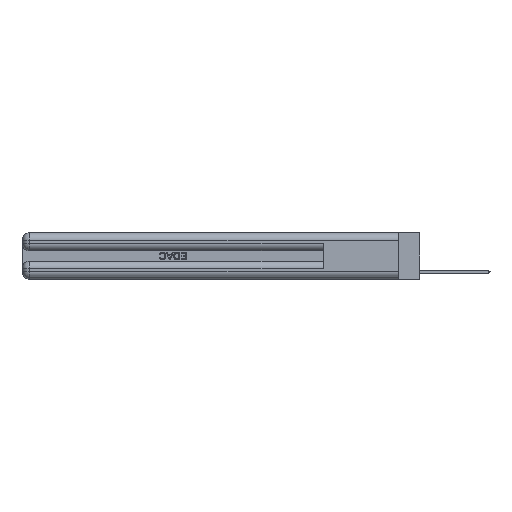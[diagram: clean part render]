
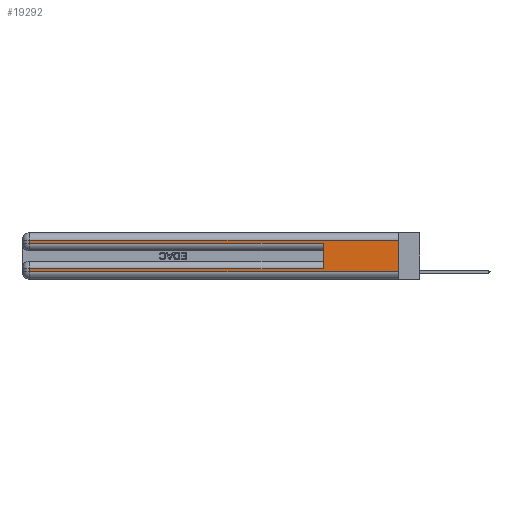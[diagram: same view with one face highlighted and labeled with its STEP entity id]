
A CAD part, left-side view. The second image highlights one B-rep face of the part: STEP entity #19292.
In plain terms, the highlighted planar face has unit normal (-1, 0, 0).
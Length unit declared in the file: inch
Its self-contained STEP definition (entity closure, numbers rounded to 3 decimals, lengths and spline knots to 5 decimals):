
#605 = VERTEX_POINT ( 'NONE', #7229 ) ;
#1070 = VECTOR ( 'NONE', #4378, 39.37008 ) ;
#1285 = LINE ( 'NONE', #17142, #4442 ) ;
#1481 = CARTESIAN_POINT ( 'NONE',  ( 0., 0.6, 0.145 ) ) ;
#1705 = CARTESIAN_POINT ( 'NONE',  ( 0., 0., 0.285 ) ) ;
#2205 = DIRECTION ( 'NONE',  ( 0., -1., 0. ) ) ;
#2462 = DIRECTION ( 'NONE',  ( 0., 0., 1. ) ) ;
#2472 = CARTESIAN_POINT ( 'NONE',  ( 0., 0., 0.31 ) ) ;
#3097 = VERTEX_POINT ( 'NONE', #30010 ) ;
#3141 = EDGE_CURVE ( 'NONE', #605, #27301, #4710, .T. ) ;
#3662 = ORIENTED_EDGE ( 'NONE', *, *, #11765, .T. ) ;
#3922 = CARTESIAN_POINT ( 'NONE',  ( 0., 2.94, 0.085 ) ) ;
#4378 = DIRECTION ( 'NONE',  ( 0., 1., 0. ) ) ;
#4442 = VECTOR ( 'NONE', #14742, 39.37008 ) ;
#4710 = LINE ( 'NONE', #27441, #1070 ) ;
#5021 = DIRECTION ( 'NONE',  ( 0., 1., 0. ) ) ;
#6286 = CARTESIAN_POINT ( 'NONE',  ( 0., 0., 0.37 ) ) ;
#6778 = VERTEX_POINT ( 'NONE', #8180 ) ;
#7229 = CARTESIAN_POINT ( 'NONE',  ( 0., 0.6, 0.085 ) ) ;
#7484 = AXIS2_PLACEMENT_3D ( 'NONE', #27236, #9114, #19537 ) ;
#7541 = ORIENTED_EDGE ( 'NONE', *, *, #27894, .T. ) ;
#7561 = LINE ( 'NONE', #2472, #8804 ) ;
#8180 = CARTESIAN_POINT ( 'NONE',  ( 0., 2.94, 0.285 ) ) ;
#8693 = CARTESIAN_POINT ( 'NONE',  ( 0., 0.6, 0.285 ) ) ;
#8804 = VECTOR ( 'NONE', #5021, 39.37008 ) ;
#9114 = DIRECTION ( 'NONE',  ( 1., 0., 0. ) ) ;
#9680 = VECTOR ( 'NONE', #14463, 39.37008 ) ;
#10110 = ORIENTED_EDGE ( 'NONE', *, *, #33695, .T. ) ;
#10632 = ORIENTED_EDGE ( 'NONE', *, *, #3141, .T. ) ;
#11725 = VERTEX_POINT ( 'NONE', #26960 ) ;
#11765 = EDGE_CURVE ( 'NONE', #28287, #6778, #12047, .T. ) ;
#12047 = LINE ( 'NONE', #19926, #14312 ) ;
#12057 = VERTEX_POINT ( 'NONE', #29638 ) ;
#12223 = DIRECTION ( 'NONE',  ( 0., 0., -1. ) ) ;
#12850 = VECTOR ( 'NONE', #2462, 39.37008 ) ;
#14312 = VECTOR ( 'NONE', #12223, 39.37008 ) ;
#14463 = DIRECTION ( 'NONE',  ( 0., 0., -1. ) ) ;
#14520 = VECTOR ( 'NONE', #2205, 39.37008 ) ;
#14742 = DIRECTION ( 'NONE',  ( 0., 0., -1. ) ) ;
#14872 = CARTESIAN_POINT ( 'NONE',  ( 0., 0., 0.06 ) ) ;
#14916 = PLANE ( 'NONE',  #7484 ) ;
#16235 = VECTOR ( 'NONE', #32496, 39.37008 ) ;
#17142 = CARTESIAN_POINT ( 'NONE',  ( 0., 2.94, 0.37 ) ) ;
#17559 = EDGE_CURVE ( 'NONE', #605, #18305, #29842, .T. ) ;
#17745 = LINE ( 'NONE', #1705, #14520 ) ;
#18138 = CARTESIAN_POINT ( 'NONE',  ( 0., 2.94, 0.31 ) ) ;
#18305 = VERTEX_POINT ( 'NONE', #8693 ) ;
#18437 = EDGE_CURVE ( 'NONE', #6778, #18305, #17745, .T. ) ;
#19088 = EDGE_LOOP ( 'NONE', ( #21956, #7541, #3662, #22763, #26544, #10632, #31064, #10110 ) ) ;
#19292 = ADVANCED_FACE ( 'NONE', ( #22783 ), #14916, .F. ) ;
#19537 = DIRECTION ( 'NONE',  ( 0., 0., -1. ) ) ;
#19926 = CARTESIAN_POINT ( 'NONE',  ( 0., 2.94, 0.37 ) ) ;
#21587 = EDGE_CURVE ( 'NONE', #12057, #11725, #27473, .T. ) ;
#21956 = ORIENTED_EDGE ( 'NONE', *, *, #21587, .F. ) ;
#22763 = ORIENTED_EDGE ( 'NONE', *, *, #18437, .T. ) ;
#22783 = FACE_OUTER_BOUND ( 'NONE', #19088, .T. ) ;
#24970 = LINE ( 'NONE', #14872, #16235 ) ;
#26544 = ORIENTED_EDGE ( 'NONE', *, *, #17559, .F. ) ;
#26960 = CARTESIAN_POINT ( 'NONE',  ( 0., 0., 0.06 ) ) ;
#27236 = CARTESIAN_POINT ( 'NONE',  ( 0., 0., 0.37 ) ) ;
#27301 = VERTEX_POINT ( 'NONE', #3922 ) ;
#27441 = CARTESIAN_POINT ( 'NONE',  ( 0., 0., 0.085 ) ) ;
#27473 = LINE ( 'NONE', #6286, #9680 ) ;
#27691 = EDGE_CURVE ( 'NONE', #27301, #3097, #1285, .T. ) ;
#27894 = EDGE_CURVE ( 'NONE', #12057, #28287, #7561, .T. ) ;
#28287 = VERTEX_POINT ( 'NONE', #18138 ) ;
#29638 = CARTESIAN_POINT ( 'NONE',  ( 0., 0., 0.31 ) ) ;
#29842 = LINE ( 'NONE', #1481, #12850 ) ;
#30010 = CARTESIAN_POINT ( 'NONE',  ( 0., 2.94, 0.06 ) ) ;
#31064 = ORIENTED_EDGE ( 'NONE', *, *, #27691, .T. ) ;
#32496 = DIRECTION ( 'NONE',  ( 0., -1., 0. ) ) ;
#33695 = EDGE_CURVE ( 'NONE', #3097, #11725, #24970, .T. ) ;
